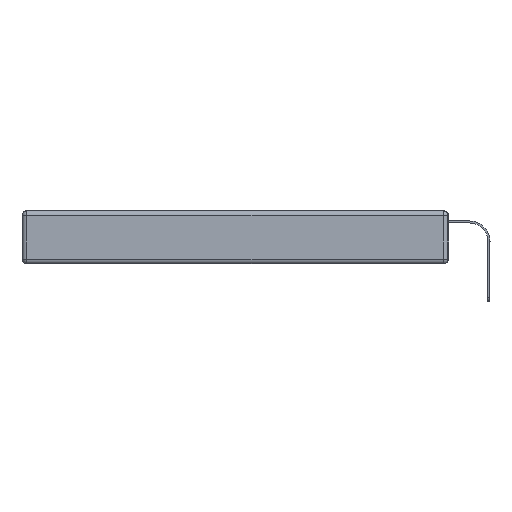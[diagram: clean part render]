
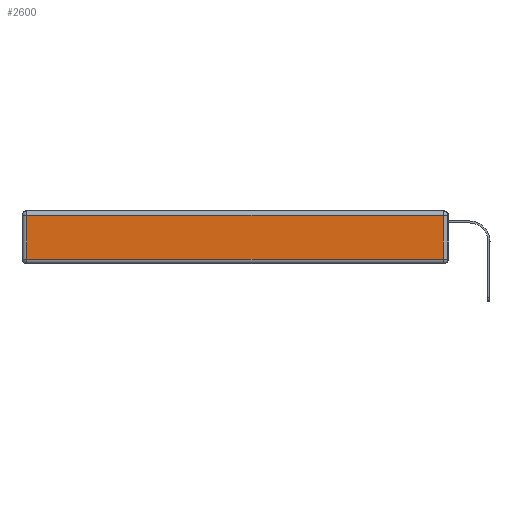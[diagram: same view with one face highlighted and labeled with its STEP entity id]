
A CAD part, left-side view. The second image highlights one B-rep face of the part: STEP entity #2600.
In plain terms, the highlighted planar face has unit normal (-1, 0, 0).
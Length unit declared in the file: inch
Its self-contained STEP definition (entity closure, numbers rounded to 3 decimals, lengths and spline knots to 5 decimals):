
#6 = VERTEX_POINT ( 'NONE', #12111 ) ;
#210 = EDGE_CURVE ( 'NONE', #9135, #7256, #20731, .T. ) ;
#1252 = EDGE_CURVE ( 'NONE', #6, #5669, #10736, .T. ) ;
#1463 = LINE ( 'NONE', #10179, #18483 ) ;
#2600 = ADVANCED_FACE ( 'NONE', ( #7414 ), #7533, .T. ) ;
#5669 = VERTEX_POINT ( 'NONE', #16366 ) ;
#6335 = EDGE_CURVE ( 'NONE', #5669, #9135, #1463, .T. ) ;
#7154 = VECTOR ( 'NONE', #9521, 39.37008 ) ;
#7256 = VERTEX_POINT ( 'NONE', #15863 ) ;
#7414 = FACE_OUTER_BOUND ( 'NONE', #9487, .T. ) ;
#7533 = PLANE ( 'NONE',  #19197 ) ;
#7951 = CARTESIAN_POINT ( 'NONE',  ( 0., 0., -0.313 ) ) ;
#8731 = EDGE_CURVE ( 'NONE', #7256, #6, #9410, .T. ) ;
#9135 = VERTEX_POINT ( 'NONE', #14321 ) ;
#9410 = LINE ( 'NONE', #19770, #7154 ) ;
#9487 = EDGE_LOOP ( 'NONE', ( #17428, #14279, #19810, #20602 ) ) ;
#9521 = DIRECTION ( 'NONE',  ( 0., 0., 1. ) ) ;
#10179 = CARTESIAN_POINT ( 'NONE',  ( 0., 2.72, -0.343 ) ) ;
#10736 = LINE ( 'NONE', #14293, #11079 ) ;
#10981 = VECTOR ( 'NONE', #19013, 39.37008 ) ;
#11079 = VECTOR ( 'NONE', #21332, 39.37008 ) ;
#12111 = CARTESIAN_POINT ( 'NONE',  ( 0., 0.03, -0.03 ) ) ;
#14279 = ORIENTED_EDGE ( 'NONE', *, *, #8731, .T. ) ;
#14293 = CARTESIAN_POINT ( 'NONE',  ( 0., 2.75, -0.03 ) ) ;
#14321 = CARTESIAN_POINT ( 'NONE',  ( 0., 2.72, -0.313 ) ) ;
#15863 = CARTESIAN_POINT ( 'NONE',  ( 0., 0.03, -0.313 ) ) ;
#16366 = CARTESIAN_POINT ( 'NONE',  ( 0., 2.72, -0.03 ) ) ;
#17195 = DIRECTION ( 'NONE',  ( 0., 0., -1. ) ) ;
#17428 = ORIENTED_EDGE ( 'NONE', *, *, #210, .T. ) ;
#17902 = DIRECTION ( 'NONE',  ( 0., 0., 1. ) ) ;
#18483 = VECTOR ( 'NONE', #17195, 39.37008 ) ;
#19013 = DIRECTION ( 'NONE',  ( 0., -1., 0. ) ) ;
#19197 = AXIS2_PLACEMENT_3D ( 'NONE', #19637, #21718, #17902 ) ;
#19637 = CARTESIAN_POINT ( 'NONE',  ( 0., 0., -0.343 ) ) ;
#19770 = CARTESIAN_POINT ( 'NONE',  ( 0., 0.03, -0.343 ) ) ;
#19810 = ORIENTED_EDGE ( 'NONE', *, *, #1252, .T. ) ;
#20602 = ORIENTED_EDGE ( 'NONE', *, *, #6335, .T. ) ;
#20731 = LINE ( 'NONE', #7951, #10981 ) ;
#21332 = DIRECTION ( 'NONE',  ( 0., 1., 0. ) ) ;
#21718 = DIRECTION ( 'NONE',  ( -1., 0., 0. ) ) ;
